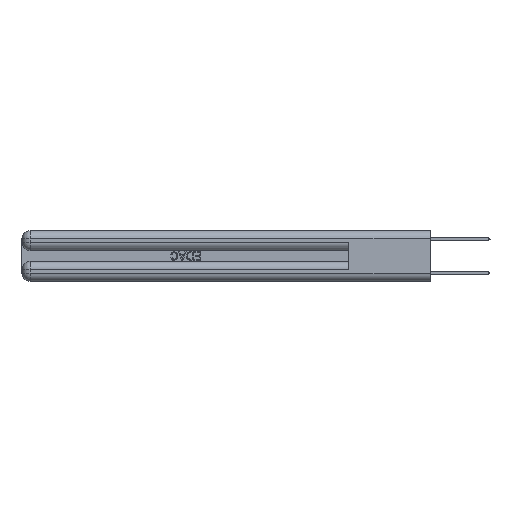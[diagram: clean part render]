
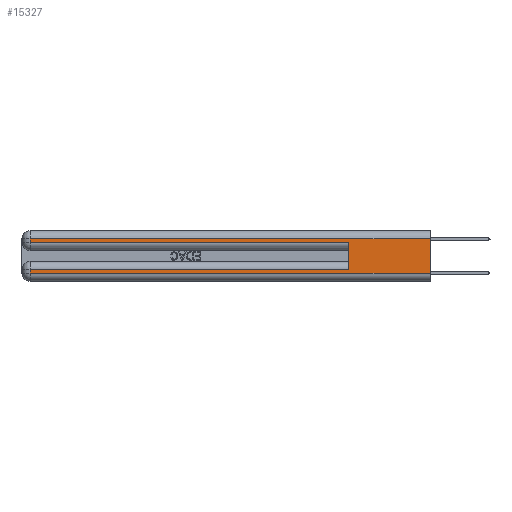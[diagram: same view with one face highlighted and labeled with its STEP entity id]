
A CAD part, left-side view. The second image highlights one B-rep face of the part: STEP entity #15327.
In plain terms, the highlighted planar face has unit normal (-1, 0, 0).
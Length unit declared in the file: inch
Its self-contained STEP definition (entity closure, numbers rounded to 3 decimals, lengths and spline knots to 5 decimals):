
#896 = VECTOR ( 'NONE', #14898, 39.37008 ) ;
#1120 = CARTESIAN_POINT ( 'NONE',  ( 0., 0., 0.06 ) ) ;
#1417 = DIRECTION ( 'NONE',  ( 0., -1., 0. ) ) ;
#1593 = LINE ( 'NONE', #22053, #896 ) ;
#2124 = ORIENTED_EDGE ( 'NONE', *, *, #20387, .T. ) ;
#2155 = EDGE_CURVE ( 'NONE', #2389, #19773, #17385, .T. ) ;
#2389 = VERTEX_POINT ( 'NONE', #18827 ) ;
#2721 = CARTESIAN_POINT ( 'NONE',  ( 0., 2.94, 0.285 ) ) ;
#3600 = CARTESIAN_POINT ( 'NONE',  ( 0., 0., 0.31 ) ) ;
#3849 = VERTEX_POINT ( 'NONE', #2721 ) ;
#3923 = DIRECTION ( 'NONE',  ( 0., -1., 0. ) ) ;
#4697 = LINE ( 'NONE', #19126, #22583 ) ;
#6954 = VECTOR ( 'NONE', #1417, 39.37008 ) ;
#7244 = VECTOR ( 'NONE', #12933, 39.37008 ) ;
#7835 = AXIS2_PLACEMENT_3D ( 'NONE', #9303, #24857, #13724 ) ;
#7951 = LINE ( 'NONE', #15388, #16582 ) ;
#7965 = VERTEX_POINT ( 'NONE', #25876 ) ;
#8034 = DIRECTION ( 'NONE',  ( 0., 0., -1. ) ) ;
#8395 = CARTESIAN_POINT ( 'NONE',  ( 0., 0., 0.285 ) ) ;
#8469 = VECTOR ( 'NONE', #8034, 39.37008 ) ;
#8654 = FACE_OUTER_BOUND ( 'NONE', #29115, .T. ) ;
#8762 = VERTEX_POINT ( 'NONE', #24462 ) ;
#9158 = EDGE_CURVE ( 'NONE', #10911, #8762, #4697, .T. ) ;
#9167 = ORIENTED_EDGE ( 'NONE', *, *, #24214, .T. ) ;
#9303 = CARTESIAN_POINT ( 'NONE',  ( 0., 0., 0.37 ) ) ;
#10063 = CARTESIAN_POINT ( 'NONE',  ( 0., 0., 0.06 ) ) ;
#10338 = DIRECTION ( 'NONE',  ( 0., 0., 1. ) ) ;
#10911 = VERTEX_POINT ( 'NONE', #14386 ) ;
#11286 = ORIENTED_EDGE ( 'NONE', *, *, #27688, .T. ) ;
#11928 = EDGE_CURVE ( 'NONE', #17063, #19773, #23845, .T. ) ;
#12684 = LINE ( 'NONE', #29032, #7244 ) ;
#12933 = DIRECTION ( 'NONE',  ( 0., 0., -1. ) ) ;
#13696 = ORIENTED_EDGE ( 'NONE', *, *, #11928, .F. ) ;
#13724 = DIRECTION ( 'NONE',  ( 0., 0., -1. ) ) ;
#13832 = PLANE ( 'NONE',  #7835 ) ;
#14386 = CARTESIAN_POINT ( 'NONE',  ( 0., 0.6, 0.085 ) ) ;
#14898 = DIRECTION ( 'NONE',  ( 0., 0., -1. ) ) ;
#15327 = ADVANCED_FACE ( 'NONE', ( #8654 ), #13832, .F. ) ;
#15388 = CARTESIAN_POINT ( 'NONE',  ( 0., 0., 0.085 ) ) ;
#16582 = VECTOR ( 'NONE', #17625, 39.37008 ) ;
#16697 = LINE ( 'NONE', #20351, #27020 ) ;
#17063 = VERTEX_POINT ( 'NONE', #3600 ) ;
#17385 = LINE ( 'NONE', #10063, #6954 ) ;
#17625 = DIRECTION ( 'NONE',  ( 0., 1., 0. ) ) ;
#18026 = DIRECTION ( 'NONE',  ( 0., 1., 0. ) ) ;
#18284 = ORIENTED_EDGE ( 'NONE', *, *, #9158, .F. ) ;
#18816 = ORIENTED_EDGE ( 'NONE', *, *, #2155, .T. ) ;
#18827 = CARTESIAN_POINT ( 'NONE',  ( 0., 2.94, 0.06 ) ) ;
#19126 = CARTESIAN_POINT ( 'NONE',  ( 0., 0.6, 0.145 ) ) ;
#19614 = CARTESIAN_POINT ( 'NONE',  ( 0., 2.94, 0.085 ) ) ;
#19773 = VERTEX_POINT ( 'NONE', #1120 ) ;
#19783 = VERTEX_POINT ( 'NONE', #19614 ) ;
#20281 = EDGE_CURVE ( 'NONE', #19783, #2389, #1593, .T. ) ;
#20351 = CARTESIAN_POINT ( 'NONE',  ( 0., 0., 0.31 ) ) ;
#20387 = EDGE_CURVE ( 'NONE', #7965, #3849, #12684, .T. ) ;
#21866 = CARTESIAN_POINT ( 'NONE',  ( 0., 0., 0.37 ) ) ;
#22053 = CARTESIAN_POINT ( 'NONE',  ( 0., 2.94, 0.37 ) ) ;
#22383 = ORIENTED_EDGE ( 'NONE', *, *, #20281, .T. ) ;
#22583 = VECTOR ( 'NONE', #10338, 39.37008 ) ;
#23845 = LINE ( 'NONE', #21866, #8469 ) ;
#24214 = EDGE_CURVE ( 'NONE', #17063, #7965, #16697, .T. ) ;
#24462 = CARTESIAN_POINT ( 'NONE',  ( 0., 0.6, 0.285 ) ) ;
#24857 = DIRECTION ( 'NONE',  ( 1., 0., 0. ) ) ;
#24897 = ORIENTED_EDGE ( 'NONE', *, *, #26847, .T. ) ;
#25876 = CARTESIAN_POINT ( 'NONE',  ( 0., 2.94, 0.31 ) ) ;
#26847 = EDGE_CURVE ( 'NONE', #10911, #19783, #7951, .T. ) ;
#26852 = VECTOR ( 'NONE', #3923, 39.37008 ) ;
#27020 = VECTOR ( 'NONE', #18026, 39.37008 ) ;
#27212 = LINE ( 'NONE', #8395, #26852 ) ;
#27688 = EDGE_CURVE ( 'NONE', #3849, #8762, #27212, .T. ) ;
#29032 = CARTESIAN_POINT ( 'NONE',  ( 0., 2.94, 0.37 ) ) ;
#29115 = EDGE_LOOP ( 'NONE', ( #13696, #9167, #2124, #11286, #18284, #24897, #22383, #18816 ) ) ;
